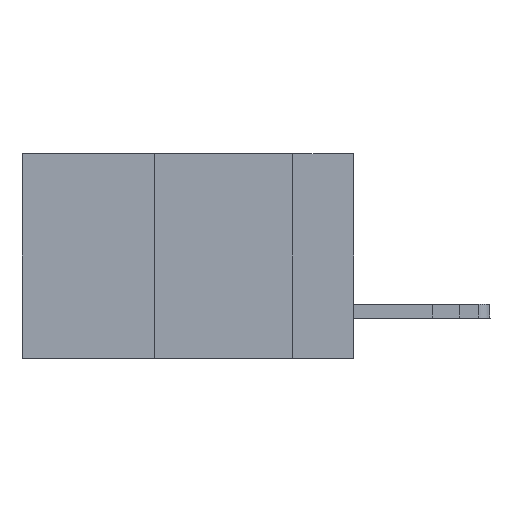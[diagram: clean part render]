
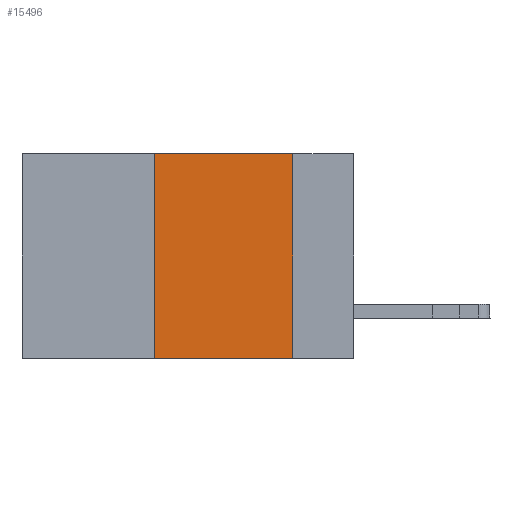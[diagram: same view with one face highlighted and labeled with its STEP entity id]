
A CAD part, left-side view. The second image highlights one B-rep face of the part: STEP entity #15496.
In plain terms, the highlighted planar face has unit normal (-1, 0, 0).
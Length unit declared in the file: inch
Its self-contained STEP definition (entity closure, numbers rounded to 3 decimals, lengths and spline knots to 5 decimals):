
#985 = DIRECTION ( 'NONE',  ( 1., 0., 0. ) ) ;
#1635 = CARTESIAN_POINT ( 'NONE',  ( 0., 0.6, -0.37 ) ) ;
#2181 = AXIS2_PLACEMENT_3D ( 'NONE', #4092, #985, #3022 ) ;
#3022 = DIRECTION ( 'NONE',  ( 0., 0., -1. ) ) ;
#3270 = LINE ( 'NONE', #12361, #16493 ) ;
#3701 = DIRECTION ( 'NONE',  ( 0., 0., -1. ) ) ;
#3928 = CARTESIAN_POINT ( 'NONE',  ( 0., 0.11, -0.37 ) ) ;
#3966 = VERTEX_POINT ( 'NONE', #3928 ) ;
#4092 = CARTESIAN_POINT ( 'NONE',  ( 0., 0.6, 0. ) ) ;
#4118 = LINE ( 'NONE', #11297, #7484 ) ;
#5294 = EDGE_CURVE ( 'NONE', #21041, #3966, #21947, .T. ) ;
#5876 = PLANE ( 'NONE',  #2181 ) ;
#6094 = VECTOR ( 'NONE', #3701, 39.37008 ) ;
#7484 = VECTOR ( 'NONE', #9613, 39.37008 ) ;
#7504 = EDGE_LOOP ( 'NONE', ( #17490, #9986, #15974, #22965 ) ) ;
#8043 = EDGE_CURVE ( 'NONE', #22885, #16380, #3270, .T. ) ;
#9568 = CARTESIAN_POINT ( 'NONE',  ( 0., 0.36, 0. ) ) ;
#9613 = DIRECTION ( 'NONE',  ( 0., -1., 0. ) ) ;
#9986 = ORIENTED_EDGE ( 'NONE', *, *, #18906, .F. ) ;
#11297 = CARTESIAN_POINT ( 'NONE',  ( 0., 0.6, 0. ) ) ;
#12361 = CARTESIAN_POINT ( 'NONE',  ( 0., 0.36, 0. ) ) ;
#14264 = DIRECTION ( 'NONE',  ( 0., 0., 1. ) ) ;
#14742 = VECTOR ( 'NONE', #21440, 39.37008 ) ;
#14923 = CARTESIAN_POINT ( 'NONE',  ( 0., 0.11, 0. ) ) ;
#15496 = ADVANCED_FACE ( 'NONE', ( #20676 ), #5876, .F. ) ;
#15974 = ORIENTED_EDGE ( 'NONE', *, *, #8043, .F. ) ;
#16380 = VERTEX_POINT ( 'NONE', #9568 ) ;
#16493 = VECTOR ( 'NONE', #14264, 39.37008 ) ;
#17188 = CARTESIAN_POINT ( 'NONE',  ( 0., 0.11, 0. ) ) ;
#17281 = CARTESIAN_POINT ( 'NONE',  ( 0., 0.36, -0.37 ) ) ;
#17490 = ORIENTED_EDGE ( 'NONE', *, *, #5294, .F. ) ;
#18766 = EDGE_CURVE ( 'NONE', #22885, #3966, #19774, .T. ) ;
#18906 = EDGE_CURVE ( 'NONE', #16380, #21041, #4118, .T. ) ;
#19774 = LINE ( 'NONE', #1635, #14742 ) ;
#20676 = FACE_OUTER_BOUND ( 'NONE', #7504, .T. ) ;
#21041 = VERTEX_POINT ( 'NONE', #17188 ) ;
#21440 = DIRECTION ( 'NONE',  ( 0., -1., 0. ) ) ;
#21947 = LINE ( 'NONE', #14923, #6094 ) ;
#22885 = VERTEX_POINT ( 'NONE', #17281 ) ;
#22965 = ORIENTED_EDGE ( 'NONE', *, *, #18766, .T. ) ;
